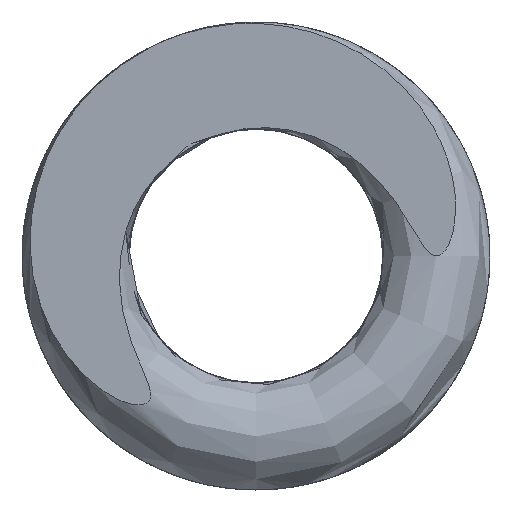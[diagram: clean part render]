
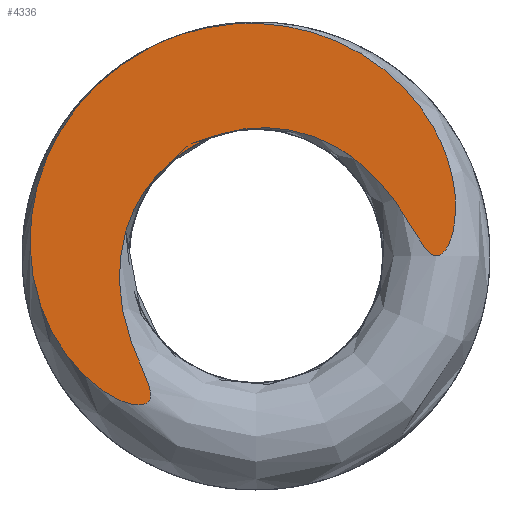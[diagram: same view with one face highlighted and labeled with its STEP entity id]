
A CAD part, front view. The second image highlights one B-rep face of the part: STEP entity #4336.
In plain terms, the highlighted planar face has unit normal (0, -1, 0).
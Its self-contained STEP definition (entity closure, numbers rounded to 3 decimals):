
#240 = ORIENTED_EDGE ( 'NONE', *, *, #4372, .T. ) ;
#554 = CARTESIAN_POINT ( 'NONE',  ( -0.945, 0.27, 0.7 ) ) ;
#576 = CARTESIAN_POINT ( 'NONE',  ( -0.685, 0.27, 0.088 ) ) ;
#1301 = CARTESIAN_POINT ( 'NONE',  ( -1.304, 0.27, -5. ) ) ;
#1542 = CARTESIAN_POINT ( 'NONE',  ( -0.429, 0.27, 0.501 ) ) ;
#1607 = CARTESIAN_POINT ( 'NONE',  ( -0.585, 0.27, -0.544 ) ) ;
#1739 = CARTESIAN_POINT ( 'NONE',  ( -0.527, 0.27, 1.056 ) ) ;
#1828 = CARTESIAN_POINT ( 'NONE',  ( -0.286, 0.27, 0.573 ) ) ;
#1964 = CARTESIAN_POINT ( 'NONE',  ( -0.548, 0.27, 0.378 ) ) ;
#2153 = ORIENTED_EDGE ( 'NONE', *, *, #3975, .T. ) ;
#2182 = CARTESIAN_POINT ( 'NONE',  ( -0.667, 0.27, -0.318 ) ) ;
#2420 = CARTESIAN_POINT ( 'NONE',  ( -0.645, 0.27, -0.395 ) ) ;
#2447 = CARTESIAN_POINT ( 'NONE',  ( -0.703, 0.27, -0.078 ) ) ;
#2499 = CARTESIAN_POINT ( 'NONE',  ( -0.601, 0.27, -0.508 ) ) ;
#2528 = B_SPLINE_CURVE_WITH_KNOTS ( 'NONE', 3,
 ( #7042, #7077, #6993, #6958, #6931, #6905, #6877, #6796, #6640, #6576, #6551, #6500, #6475, #6422, #6412, #6393, #6384, #6358, #6331, #6305, #6255, #6229, #6202, #6175, #6123, #6073, #6048, #6025, #5933, #5906, #5880, #5853 ),
 .UNSPECIFIED., .F., .F.,
 ( 4, 2, 2, 2, 2, 2, 2, 2, 2, 2, 2, 2, 2, 2, 2, 4 ),
 ( 0.006, 0.007, 0.007, 0.007, 0.007, 0.008, 0.008, 0.008, 0.008, 0.008, 0.008, 0.008, 0.009, 0.009, 0.01, 0.01 ),
 .UNSPECIFIED. ) ;
#2631 = AXIS2_PLACEMENT_3D ( 'NONE', #1301, #7153, #7127 ) ;
#2749 = CARTESIAN_POINT ( 'NONE',  ( -0.553, 0.27, -0.618 ) ) ;
#2991 = CARTESIAN_POINT ( 'NONE',  ( -0.534, 0.27, -0.655 ) ) ;
#3113 = CARTESIAN_POINT ( 'NONE',  ( -0.527, 0.27, 1.056 ) ) ;
#3230 = CARTESIAN_POINT ( 'NONE',  ( -0.8, 0.27, -0.666 ) ) ;
#3257 = CARTESIAN_POINT ( 'NONE',  ( -0.542, 0.27, -0.735 ) ) ;
#3311 = CARTESIAN_POINT ( 'NONE',  ( -0.532, 0.27, -0.706 ) ) ;
#3374 = CARTESIAN_POINT ( 'NONE',  ( -1.087, 0.27, -0.286 ) ) ;
#3412 = CARTESIAN_POINT ( 'NONE',  ( -0.668, 0.27, 0.985 ) ) ;
#3458 = CARTESIAN_POINT ( 'NONE',  ( -0.533, 0.27, -0.716 ) ) ;
#3710 = CARTESIAN_POINT ( 'NONE',  ( -0.55, 0.27, -0.742 ) ) ;
#3764 = CARTESIAN_POINT ( 'NONE',  ( -0.696, 0.27, -0.725 ) ) ;
#3792 = CARTESIAN_POINT ( 'NONE',  ( -0.599, 0.27, -0.752 ) ) ;
#3847 = CARTESIAN_POINT ( 'NONE',  ( -0.659, 0.27, -0.742 ) ) ;
#3938 = CARTESIAN_POINT ( 'NONE',  ( -1.141, 0.27, 0.027 ) ) ;
#3958 = CARTESIAN_POINT ( 'NONE',  ( -1.137, 0.27, 0.184 ) ) ;
#3975 = EDGE_CURVE ( 'NONE', #7089, #4276, #5108, .T. ) ;
#3986 = CARTESIAN_POINT ( 'NONE',  ( -0.862, 0.27, -0.612 ) ) ;
#4015 = CARTESIAN_POINT ( 'NONE',  ( -1.017, 0.27, -0.434 ) ) ;
#4044 = CARTESIAN_POINT ( 'NONE',  ( -1.135, 0.27, -0.054 ) ) ;
#4135 = CARTESIAN_POINT ( 'NONE',  ( -1.126, 0.27, 0.263 ) ) ;
#4260 = FACE_OUTER_BOUND ( 'NONE', #7668, .T. ) ;
#4276 = VERTEX_POINT ( 'NONE', #4731 ) ;
#4312 = CARTESIAN_POINT ( 'NONE',  ( -1.087, 0.27, 0.418 ) ) ;
#4336 = ADVANCED_FACE ( 'NONE', ( #4260 ), #7293, .F. ) ;
#4372 = EDGE_CURVE ( 'NONE', #4276, #7089, #2528, .T. ) ;
#4584 = CARTESIAN_POINT ( 'NONE',  ( -0.989, 0.27, 0.632 ) ) ;
#4731 = CARTESIAN_POINT ( 'NONE',  ( -0.286, 0.27, 0.573 ) ) ;
#4983 = CARTESIAN_POINT ( 'NONE',  ( -0.578, 0.27, -0.753 ) ) ;
#5108 = B_SPLINE_CURVE_WITH_KNOTS ( 'NONE', 3,
 ( #1739, #3412, #5684, #554, #4584, #6823, #4312, #4135, #3958, #3938, #4044, #3374, #4015, #3986, #3230, #3764, #3847, #3792, #4983, #3710, #3257, #3458, #3311, #2991, #2749, #1607, #2499, #2420, #2182, #2447, #576, #1964, #1542, #1828 ),
 .UNSPECIFIED., .F., .F.,
 ( 4, 2, 2, 2, 2, 2, 2, 2, 2, 2, 2, 2, 2, 2, 2, 2, 4 ),
 ( 0.002, 0.003, 0.003, 0.003, 0.004, 0.004, 0.004, 0.005, 0.005, 0.005, 0.005, 0.005, 0.005, 0.005, 0.005, 0.006, 0.006 ),
 .UNSPECIFIED. ) ;
#5684 = CARTESIAN_POINT ( 'NONE',  ( -0.795, 0.27, 0.884 ) ) ;
#5853 = CARTESIAN_POINT ( 'NONE',  ( -0.527, 0.27, 1.056 ) ) ;
#5880 = CARTESIAN_POINT ( 'NONE',  ( -0.387, 0.27, 1.126 ) ) ;
#5906 = CARTESIAN_POINT ( 'NONE',  ( -0.231, 0.27, 1.166 ) ) ;
#5933 = CARTESIAN_POINT ( 'NONE',  ( 0.084, 0.27, 1.179 ) ) ;
#6025 = CARTESIAN_POINT ( 'NONE',  ( 0.243, 0.27, 1.151 ) ) ;
#6048 = CARTESIAN_POINT ( 'NONE',  ( 0.535, 0.27, 1.03 ) ) ;
#6073 = CARTESIAN_POINT ( 'NONE',  ( 0.667, 0.27, 0.937 ) ) ;
#6123 = CARTESIAN_POINT ( 'NONE',  ( 0.877, 0.27, 0.703 ) ) ;
#6175 = CARTESIAN_POINT ( 'NONE',  ( 0.956, 0.27, 0.558 ) ) ;
#6202 = CARTESIAN_POINT ( 'NONE',  ( 1.006, 0.27, 0.327 ) ) ;
#6229 = CARTESIAN_POINT ( 'NONE',  ( 1.012, 0.27, 0.247 ) ) ;
#6255 = CARTESIAN_POINT ( 'NONE',  ( 0.996, 0.27, 0.129 ) ) ;
#6305 = CARTESIAN_POINT ( 'NONE',  ( 0.987, 0.27, 0.089 ) ) ;
#6331 = CARTESIAN_POINT ( 'NONE',  ( 0.961, 0.27, 0.036 ) ) ;
#6358 = CARTESIAN_POINT ( 'NONE',  ( 0.95, 0.27, 0.018 ) ) ;
#6384 = CARTESIAN_POINT ( 'NONE',  ( 0.924, 0.27, 0.002 ) ) ;
#6393 = CARTESIAN_POINT ( 'NONE',  ( 0.914, 0.27, -0.001 ) ) ;
#6412 = CARTESIAN_POINT ( 'NONE',  ( 0.894, 0.27, 0.002 ) ) ;
#6422 = CARTESIAN_POINT ( 'NONE',  ( 0.885, 0.27, 0.008 ) ) ;
#6475 = CARTESIAN_POINT ( 'NONE',  ( 0.846, 0.27, 0.039 ) ) ;
#6500 = CARTESIAN_POINT ( 'NONE',  ( 0.827, 0.27, 0.076 ) ) ;
#6551 = CARTESIAN_POINT ( 'NONE',  ( 0.786, 0.27, 0.145 ) ) ;
#6576 = CARTESIAN_POINT ( 'NONE',  ( 0.765, 0.27, 0.18 ) ) ;
#6640 = CARTESIAN_POINT ( 'NONE',  ( 0.7, 0.27, 0.282 ) ) ;
#6796 = CARTESIAN_POINT ( 'NONE',  ( 0.651, 0.27, 0.346 ) ) ;
#6823 = CARTESIAN_POINT ( 'NONE',  ( -1.059, 0.27, 0.491 ) ) ;
#6877 = CARTESIAN_POINT ( 'NONE',  ( 0.54, 0.27, 0.459 ) ) ;
#6905 = CARTESIAN_POINT ( 'NONE',  ( 0.476, 0.27, 0.51 ) ) ;
#6931 = CARTESIAN_POINT ( 'NONE',  ( 0.337, 0.27, 0.588 ) ) ;
#6958 = CARTESIAN_POINT ( 'NONE',  ( 0.26, 0.27, 0.617 ) ) ;
#6993 = CARTESIAN_POINT ( 'NONE',  ( 0.025, 0.27, 0.665 ) ) ;
#7042 = CARTESIAN_POINT ( 'NONE',  ( -0.286, 0.27, 0.573 ) ) ;
#7077 = CARTESIAN_POINT ( 'NONE',  ( -0.143, 0.27, 0.644 ) ) ;
#7089 = VERTEX_POINT ( 'NONE', #3113 ) ;
#7127 = DIRECTION ( 'NONE',  ( -1., 0., 0. ) ) ;
#7153 = DIRECTION ( 'NONE',  ( 0., 1., 0. ) ) ;
#7293 = PLANE ( 'NONE',  #2631 ) ;
#7668 = EDGE_LOOP ( 'NONE', ( #2153, #240 ) ) ;
